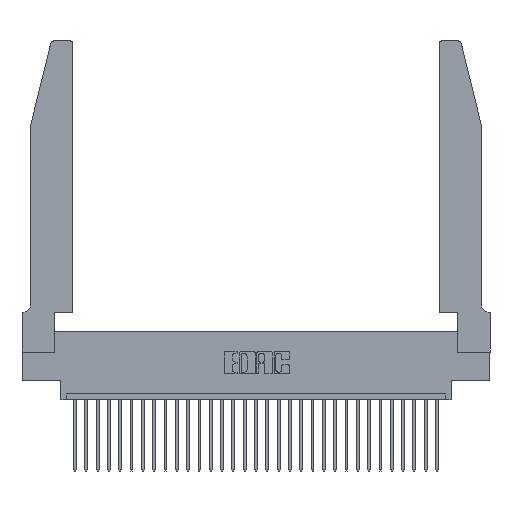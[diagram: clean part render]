
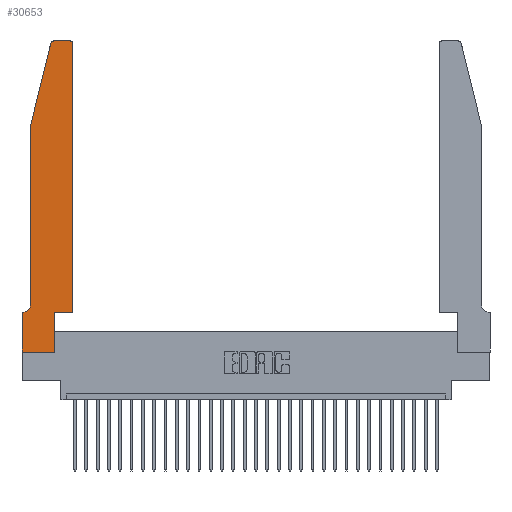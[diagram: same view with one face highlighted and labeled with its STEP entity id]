
A CAD part, top view. The second image highlights one B-rep face of the part: STEP entity #30653.
In plain terms, the highlighted planar face has unit normal (0, 0, 1).
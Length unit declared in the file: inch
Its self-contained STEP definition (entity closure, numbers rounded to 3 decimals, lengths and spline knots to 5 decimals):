
#55 = DIRECTION ( 'NONE',  ( 0., 0., 1. ) ) ;
#765 = ORIENTED_EDGE ( 'NONE', *, *, #30315, .T. ) ;
#824 = LINE ( 'NONE', #2398, #27740 ) ;
#995 = DIRECTION ( 'NONE',  ( 1., 0., 0. ) ) ;
#1734 = DIRECTION ( 'NONE',  ( 0., -1., 0. ) ) ;
#1981 = CARTESIAN_POINT ( 'NONE',  ( 0.0055, 0.42, 0.37 ) ) ;
#2348 = ORIENTED_EDGE ( 'NONE', *, *, #16467, .T. ) ;
#2398 = CARTESIAN_POINT ( 'NONE',  ( 0.4505, 0.35, 0.37 ) ) ;
#2474 = ORIENTED_EDGE ( 'NONE', *, *, #19401, .T. ) ;
#2586 = AXIS2_PLACEMENT_3D ( 'NONE', #15134, #24797, #995 ) ;
#3550 = VERTEX_POINT ( 'NONE', #11962 ) ;
#3556 = VECTOR ( 'NONE', #28977, 39.37008 ) ;
#3654 = LINE ( 'NONE', #11864, #9906 ) ;
#4086 = EDGE_CURVE ( 'NONE', #21629, #21571, #14377, .T. ) ;
#4486 = DIRECTION ( 'NONE',  ( 0., 0., -1. ) ) ;
#4858 = DIRECTION ( 'NONE',  ( 0., 0., 1. ) ) ;
#5643 = VERTEX_POINT ( 'NONE', #15402 ) ;
#5830 = ORIENTED_EDGE ( 'NONE', *, *, #6615, .T. ) ;
#5839 = CIRCLE ( 'NONE', #14094, 0.03 ) ;
#6021 = CARTESIAN_POINT ( 'NONE',  ( 0.4505, 2.72, 0.37 ) ) ;
#6040 = EDGE_CURVE ( 'NONE', #6734, #5643, #26591, .T. ) ;
#6549 = EDGE_CURVE ( 'NONE', #21571, #8464, #13464, .T. ) ;
#6615 = EDGE_CURVE ( 'NONE', #30332, #24475, #8205, .T. ) ;
#6734 = VERTEX_POINT ( 'NONE', #12769 ) ;
#6970 = CARTESIAN_POINT ( 'NONE',  ( 0.4205, 2.75, 0.37 ) ) ;
#7118 = AXIS2_PLACEMENT_3D ( 'NONE', #1981, #4486, #21046 ) ;
#7229 = DIRECTION ( 'NONE',  ( 1., 0., 0. ) ) ;
#7350 = CARTESIAN_POINT ( 'NONE',  ( 0.4505, 0.35, 0.37 ) ) ;
#7418 = CARTESIAN_POINT ( 'NONE',  ( 0.2605, 2.75, 0.37 ) ) ;
#8205 = LINE ( 'NONE', #7350, #11951 ) ;
#8464 = VERTEX_POINT ( 'NONE', #13826 ) ;
#8576 = CIRCLE ( 'NONE', #9288, 0.03 ) ;
#9127 = CARTESIAN_POINT ( 'NONE',  ( 0.0755, 0.42, 0.37 ) ) ;
#9288 = AXIS2_PLACEMENT_3D ( 'NONE', #28551, #4858, #14207 ) ;
#9906 = VECTOR ( 'NONE', #19823, 39.37008 ) ;
#10136 = CARTESIAN_POINT ( 'NONE',  ( 0.2865, 0.35, 0.37 ) ) ;
#10159 = CARTESIAN_POINT ( 'NONE',  ( 0.25487, 2.72718, 0.37 ) ) ;
#10401 = ORIENTED_EDGE ( 'NONE', *, *, #6040, .T. ) ;
#10423 = LINE ( 'NONE', #13762, #30648 ) ;
#11338 = LINE ( 'NONE', #10136, #3556 ) ;
#11624 = VECTOR ( 'NONE', #13179, 39.37008 ) ;
#11864 = CARTESIAN_POINT ( 'NONE',  ( 0.0755, 2., 0.37 ) ) ;
#11951 = VECTOR ( 'NONE', #26693, 39.37008 ) ;
#11962 = CARTESIAN_POINT ( 'NONE',  ( 0.2865, 0., 0.37 ) ) ;
#12690 = EDGE_LOOP ( 'NONE', ( #18624, #18040, #18855, #25509, #29717, #2348, #10401, #21626, #12715, #2474, #5830, #765 ) ) ;
#12715 = ORIENTED_EDGE ( 'NONE', *, *, #18273, .T. ) ;
#12769 = CARTESIAN_POINT ( 'NONE',  ( 0., 0.35, 0.37 ) ) ;
#13179 = DIRECTION ( 'NONE',  ( 0., -1., 0. ) ) ;
#13464 = CIRCLE ( 'NONE', #7118, 0.07 ) ;
#13577 = CARTESIAN_POINT ( 'NONE',  ( 0.0755, 0.35, 0.37 ) ) ;
#13762 = CARTESIAN_POINT ( 'NONE',  ( 0., 0., 0.37 ) ) ;
#13826 = CARTESIAN_POINT ( 'NONE',  ( 0.0055, 0.35, 0.37 ) ) ;
#14094 = AXIS2_PLACEMENT_3D ( 'NONE', #19272, #55, #21250 ) ;
#14207 = DIRECTION ( 'NONE',  ( 1., 0., 0. ) ) ;
#14377 = LINE ( 'NONE', #20084, #22624 ) ;
#15134 = CARTESIAN_POINT ( 'NONE',  ( 0., 0.35, 0.37 ) ) ;
#15402 = CARTESIAN_POINT ( 'NONE',  ( 0., 0., 0.37 ) ) ;
#15995 = DIRECTION ( 'NONE',  ( -1., 0., 0. ) ) ;
#16381 = DIRECTION ( 'NONE',  ( 1., 0., 0. ) ) ;
#16467 = EDGE_CURVE ( 'NONE', #8464, #6734, #23016, .T. ) ;
#18040 = ORIENTED_EDGE ( 'NONE', *, *, #20311, .T. ) ;
#18273 = EDGE_CURVE ( 'NONE', #3550, #26158, #11338, .T. ) ;
#18624 = ORIENTED_EDGE ( 'NONE', *, *, #19482, .T. ) ;
#18855 = ORIENTED_EDGE ( 'NONE', *, *, #23399, .T. ) ;
#19272 = CARTESIAN_POINT ( 'NONE',  ( 0.4205, 2.72, 0.37 ) ) ;
#19401 = EDGE_CURVE ( 'NONE', #26158, #30332, #824, .T. ) ;
#19482 = EDGE_CURVE ( 'NONE', #24052, #25315, #19865, .T. ) ;
#19823 = DIRECTION ( 'NONE',  ( -0.239, -0.971, 0. ) ) ;
#19865 = LINE ( 'NONE', #7418, #25495 ) ;
#20016 = FACE_OUTER_BOUND ( 'NONE', #12690, .T. ) ;
#20084 = CARTESIAN_POINT ( 'NONE',  ( 0.0755, 2., 0.37 ) ) ;
#20311 = EDGE_CURVE ( 'NONE', #25315, #25853, #8576, .T. ) ;
#20597 = EDGE_CURVE ( 'NONE', #5643, #3550, #10423, .T. ) ;
#21046 = DIRECTION ( 'NONE',  ( -1., 0., 0. ) ) ;
#21250 = DIRECTION ( 'NONE',  ( 1., 0., 0. ) ) ;
#21571 = VERTEX_POINT ( 'NONE', #9127 ) ;
#21626 = ORIENTED_EDGE ( 'NONE', *, *, #20597, .T. ) ;
#21629 = VERTEX_POINT ( 'NONE', #28165 ) ;
#21642 = CARTESIAN_POINT ( 'NONE',  ( 0.4505, 0.35, 0.37 ) ) ;
#21943 = DIRECTION ( 'NONE',  ( -1., 0., 0. ) ) ;
#22590 = PLANE ( 'NONE',  #2586 ) ;
#22624 = VECTOR ( 'NONE', #1734, 39.37008 ) ;
#23016 = LINE ( 'NONE', #13577, #23766 ) ;
#23399 = EDGE_CURVE ( 'NONE', #25853, #21629, #3654, .T. ) ;
#23766 = VECTOR ( 'NONE', #15995, 39.37008 ) ;
#24052 = VERTEX_POINT ( 'NONE', #6970 ) ;
#24187 = CARTESIAN_POINT ( 'NONE',  ( 0., 0., 0.37 ) ) ;
#24475 = VERTEX_POINT ( 'NONE', #6021 ) ;
#24797 = DIRECTION ( 'NONE',  ( 0., 0., 1. ) ) ;
#25315 = VERTEX_POINT ( 'NONE', #28746 ) ;
#25353 = CARTESIAN_POINT ( 'NONE',  ( 0.2865, 0.35, 0.37 ) ) ;
#25495 = VECTOR ( 'NONE', #21943, 39.37008 ) ;
#25509 = ORIENTED_EDGE ( 'NONE', *, *, #4086, .T. ) ;
#25853 = VERTEX_POINT ( 'NONE', #10159 ) ;
#26158 = VERTEX_POINT ( 'NONE', #25353 ) ;
#26591 = LINE ( 'NONE', #24187, #11624 ) ;
#26693 = DIRECTION ( 'NONE',  ( 0., 1., 0. ) ) ;
#27740 = VECTOR ( 'NONE', #7229, 39.37008 ) ;
#28165 = CARTESIAN_POINT ( 'NONE',  ( 0.0755, 2., 0.37 ) ) ;
#28551 = CARTESIAN_POINT ( 'NONE',  ( 0.284, 2.72, 0.37 ) ) ;
#28746 = CARTESIAN_POINT ( 'NONE',  ( 0.284, 2.75, 0.37 ) ) ;
#28977 = DIRECTION ( 'NONE',  ( 0., 1., 0. ) ) ;
#29717 = ORIENTED_EDGE ( 'NONE', *, *, #6549, .T. ) ;
#30315 = EDGE_CURVE ( 'NONE', #24475, #24052, #5839, .T. ) ;
#30332 = VERTEX_POINT ( 'NONE', #21642 ) ;
#30648 = VECTOR ( 'NONE', #16381, 39.37008 ) ;
#30653 = ADVANCED_FACE ( 'NONE', ( #20016 ), #22590, .T. ) ;
